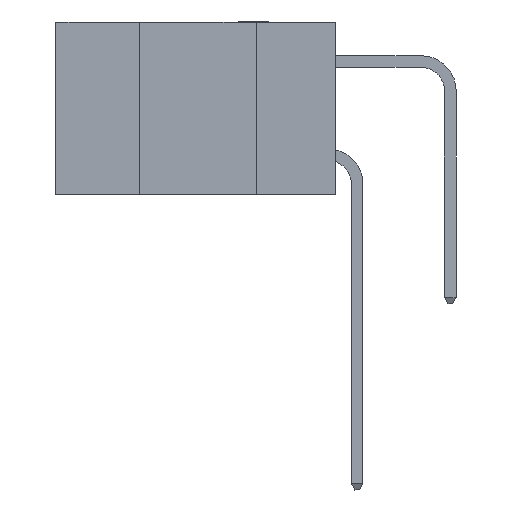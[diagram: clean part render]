
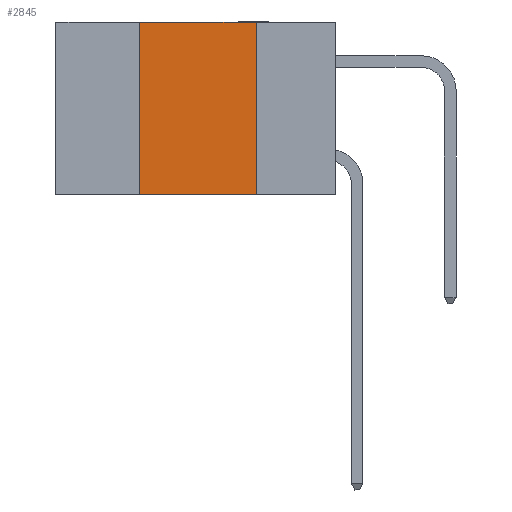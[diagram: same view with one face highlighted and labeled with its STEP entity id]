
A CAD part, left-side view. The second image highlights one B-rep face of the part: STEP entity #2845.
In plain terms, the highlighted planar face has unit normal (-1, 0, 0).
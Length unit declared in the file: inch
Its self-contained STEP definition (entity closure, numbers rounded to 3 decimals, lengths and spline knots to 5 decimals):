
#768 = CARTESIAN_POINT ( 'NONE',  ( 0., 0.17, -0.37 ) ) ;
#777 = AXIS2_PLACEMENT_3D ( 'NONE', #18997, #13994, #2370 ) ;
#1207 = VECTOR ( 'NONE', #7284, 39.37008 ) ;
#1242 = CARTESIAN_POINT ( 'NONE',  ( 0., 0.6, -0.37 ) ) ;
#1422 = EDGE_LOOP ( 'NONE', ( #10558, #10961, #12701, #16632 ) ) ;
#1453 = VERTEX_POINT ( 'NONE', #5424 ) ;
#2014 = LINE ( 'NONE', #4659, #2264 ) ;
#2262 = FACE_OUTER_BOUND ( 'NONE', #1422, .T. ) ;
#2264 = VECTOR ( 'NONE', #13040, 39.37008 ) ;
#2370 = DIRECTION ( 'NONE',  ( 0., 0., -1. ) ) ;
#2377 = EDGE_CURVE ( 'NONE', #19041, #1453, #19482, .T. ) ;
#2845 = ADVANCED_FACE ( 'NONE', ( #2262 ), #10487, .F. ) ;
#3678 = CARTESIAN_POINT ( 'NONE',  ( 0., 0.17, 0. ) ) ;
#3831 = EDGE_CURVE ( 'NONE', #18148, #7913, #21094, .T. ) ;
#3918 = CARTESIAN_POINT ( 'NONE',  ( 0., 0.42, 0. ) ) ;
#4029 = CARTESIAN_POINT ( 'NONE',  ( 0., 0.17, 0. ) ) ;
#4659 = CARTESIAN_POINT ( 'NONE',  ( 0., 0.6, 0. ) ) ;
#5424 = CARTESIAN_POINT ( 'NONE',  ( 0., 0.42, 0. ) ) ;
#7284 = DIRECTION ( 'NONE',  ( 0., 0., 1. ) ) ;
#7913 = VERTEX_POINT ( 'NONE', #768 ) ;
#10223 = CARTESIAN_POINT ( 'NONE',  ( 0., 0.42, -0.37 ) ) ;
#10487 = PLANE ( 'NONE',  #777 ) ;
#10558 = ORIENTED_EDGE ( 'NONE', *, *, #3831, .F. ) ;
#10961 = ORIENTED_EDGE ( 'NONE', *, *, #16762, .F. ) ;
#11644 = VECTOR ( 'NONE', #12936, 39.37008 ) ;
#12701 = ORIENTED_EDGE ( 'NONE', *, *, #2377, .F. ) ;
#12936 = DIRECTION ( 'NONE',  ( 0., -1., 0. ) ) ;
#13040 = DIRECTION ( 'NONE',  ( 0., -1., 0. ) ) ;
#13994 = DIRECTION ( 'NONE',  ( 1., 0., 0. ) ) ;
#15054 = LINE ( 'NONE', #1242, #11644 ) ;
#16632 = ORIENTED_EDGE ( 'NONE', *, *, #17635, .T. ) ;
#16762 = EDGE_CURVE ( 'NONE', #1453, #18148, #2014, .T. ) ;
#17095 = DIRECTION ( 'NONE',  ( 0., 0., -1. ) ) ;
#17635 = EDGE_CURVE ( 'NONE', #19041, #7913, #15054, .T. ) ;
#18148 = VERTEX_POINT ( 'NONE', #4029 ) ;
#18997 = CARTESIAN_POINT ( 'NONE',  ( 0., 0.6, 0. ) ) ;
#19041 = VERTEX_POINT ( 'NONE', #10223 ) ;
#19482 = LINE ( 'NONE', #3918, #1207 ) ;
#20837 = VECTOR ( 'NONE', #17095, 39.37008 ) ;
#21094 = LINE ( 'NONE', #3678, #20837 ) ;
